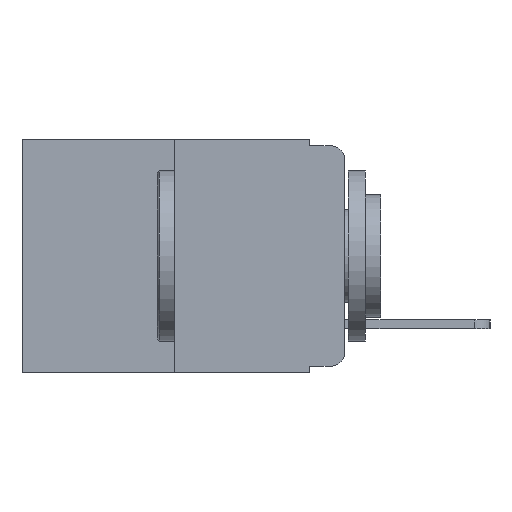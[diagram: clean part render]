
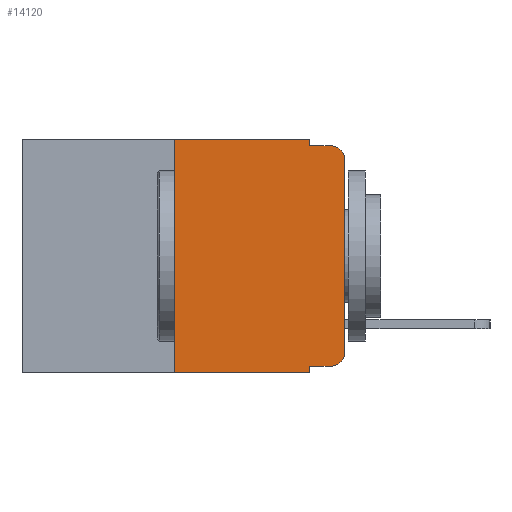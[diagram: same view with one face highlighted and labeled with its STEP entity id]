
A CAD part, left-side view. The second image highlights one B-rep face of the part: STEP entity #14120.
In plain terms, the highlighted planar face has unit normal (-1, 0, 0).
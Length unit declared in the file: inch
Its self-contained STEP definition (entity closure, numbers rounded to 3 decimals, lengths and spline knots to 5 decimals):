
#220 = AXIS2_PLACEMENT_3D ( 'NONE', #4102, #19524, #14592 ) ;
#433 = EDGE_LOOP ( 'NONE', ( #13091, #13113, #14780, #15248, #15609, #15630, #15636, #15817, #17762, #18595 ) ) ;
#1052 = VECTOR ( 'NONE', #4114, 39.37008 ) ;
#1091 = LINE ( 'NONE', #9057, #9512 ) ;
#1146 = CARTESIAN_POINT ( 'NONE',  ( 0., 0.25, -0.343 ) ) ;
#1528 = CIRCLE ( 'NONE', #2334, 0.02 ) ;
#1837 = CARTESIAN_POINT ( 'NONE',  ( 0., 0.051, 0. ) ) ;
#1863 = CARTESIAN_POINT ( 'NONE',  ( 0., 0., -0.03 ) ) ;
#1942 = LINE ( 'NONE', #18337, #5349 ) ;
#1950 = VERTEX_POINT ( 'NONE', #1146 ) ;
#2334 = AXIS2_PLACEMENT_3D ( 'NONE', #9263, #20120, #10343 ) ;
#3716 = EDGE_CURVE ( 'NONE', #14727, #7872, #1528, .T. ) ;
#3722 = DIRECTION ( 'NONE',  ( 0., 0., 1. ) ) ;
#3765 = CARTESIAN_POINT ( 'NONE',  ( 0., 0.02, -0.03 ) ) ;
#4102 = CARTESIAN_POINT ( 'NONE',  ( 0., 0.473, 0. ) ) ;
#4114 = DIRECTION ( 'NONE',  ( 0., -1., 0. ) ) ;
#4340 = DIRECTION ( 'NONE',  ( 0., 0., 1. ) ) ;
#4721 = FACE_OUTER_BOUND ( 'NONE', #433, .T. ) ;
#5335 = VECTOR ( 'NONE', #20934, 39.37008 ) ;
#5349 = VECTOR ( 'NONE', #21442, 39.37008 ) ;
#5462 = DIRECTION ( 'NONE',  ( 0., 0., -1. ) ) ;
#5794 = VERTEX_POINT ( 'NONE', #7338 ) ;
#5984 = EDGE_CURVE ( 'NONE', #5794, #14727, #1942, .T. ) ;
#7113 = EDGE_CURVE ( 'NONE', #5794, #13828, #18581, .T. ) ;
#7292 = DIRECTION ( 'NONE',  ( 0., -1., 0. ) ) ;
#7338 = CARTESIAN_POINT ( 'NONE',  ( 0., 0.051, -0.333 ) ) ;
#7716 = EDGE_CURVE ( 'NONE', #17515, #17455, #20288, .T. ) ;
#7872 = VERTEX_POINT ( 'NONE', #10326 ) ;
#8249 = EDGE_CURVE ( 'NONE', #1950, #17515, #1091, .T. ) ;
#8322 = LINE ( 'NONE', #14143, #16619 ) ;
#8709 = CARTESIAN_POINT ( 'NONE',  ( 0., 0.473, 0. ) ) ;
#9057 = CARTESIAN_POINT ( 'NONE',  ( 0., 0.25, 0. ) ) ;
#9191 = PLANE ( 'NONE',  #220 ) ;
#9263 = CARTESIAN_POINT ( 'NONE',  ( 0., 0.02, -0.313 ) ) ;
#9285 = VECTOR ( 'NONE', #3722, 39.37008 ) ;
#9380 = EDGE_CURVE ( 'NONE', #17455, #13485, #13062, .T. ) ;
#9401 = DIRECTION ( 'NONE',  ( 0., 0., -1. ) ) ;
#9512 = VECTOR ( 'NONE', #4340, 39.37008 ) ;
#10326 = CARTESIAN_POINT ( 'NONE',  ( 0., 0., -0.313 ) ) ;
#10343 = DIRECTION ( 'NONE',  ( 0., 0., -1. ) ) ;
#10504 = EDGE_CURVE ( 'NONE', #13485, #17508, #8322, .T. ) ;
#11599 = EDGE_CURVE ( 'NONE', #18146, #17508, #17863, .T. ) ;
#11746 = CARTESIAN_POINT ( 'NONE',  ( 0., 0.051, -0.343 ) ) ;
#11927 = CARTESIAN_POINT ( 'NONE',  ( 0., 0.02, -0.01 ) ) ;
#12545 = DIRECTION ( 'NONE',  ( 0., -1., 0. ) ) ;
#12707 = EDGE_CURVE ( 'NONE', #7872, #18146, #18064, .T. ) ;
#12728 = CARTESIAN_POINT ( 'NONE',  ( 0., 0.051, 0. ) ) ;
#13062 = LINE ( 'NONE', #12728, #21176 ) ;
#13091 = ORIENTED_EDGE ( 'NONE', *, *, #12707, .T. ) ;
#13113 = ORIENTED_EDGE ( 'NONE', *, *, #11599, .T. ) ;
#13485 = VERTEX_POINT ( 'NONE', #14015 ) ;
#13753 = CARTESIAN_POINT ( 'NONE',  ( 0., 0., 0. ) ) ;
#13828 = VERTEX_POINT ( 'NONE', #11746 ) ;
#14015 = CARTESIAN_POINT ( 'NONE',  ( 0., 0.051, -0.01 ) ) ;
#14120 = ADVANCED_FACE ( 'NONE', ( #4721 ), #9191, .F. ) ;
#14143 = CARTESIAN_POINT ( 'NONE',  ( 0., 0.051, -0.01 ) ) ;
#14400 = LINE ( 'NONE', #20592, #1052 ) ;
#14537 = AXIS2_PLACEMENT_3D ( 'NONE', #3765, #15445, #5462 ) ;
#14592 = DIRECTION ( 'NONE',  ( 0., 0., -1. ) ) ;
#14727 = VERTEX_POINT ( 'NONE', #19425 ) ;
#14780 = ORIENTED_EDGE ( 'NONE', *, *, #10504, .F. ) ;
#15020 = CARTESIAN_POINT ( 'NONE',  ( 0., 0.051, 0. ) ) ;
#15248 = ORIENTED_EDGE ( 'NONE', *, *, #9380, .F. ) ;
#15445 = DIRECTION ( 'NONE',  ( -1., 0., 0. ) ) ;
#15609 = ORIENTED_EDGE ( 'NONE', *, *, #7716, .F. ) ;
#15630 = ORIENTED_EDGE ( 'NONE', *, *, #8249, .F. ) ;
#15636 = ORIENTED_EDGE ( 'NONE', *, *, #18884, .T. ) ;
#15817 = ORIENTED_EDGE ( 'NONE', *, *, #7113, .F. ) ;
#16619 = VECTOR ( 'NONE', #12545, 39.37008 ) ;
#17455 = VERTEX_POINT ( 'NONE', #15020 ) ;
#17508 = VERTEX_POINT ( 'NONE', #11927 ) ;
#17515 = VERTEX_POINT ( 'NONE', #19990 ) ;
#17762 = ORIENTED_EDGE ( 'NONE', *, *, #5984, .T. ) ;
#17863 = CIRCLE ( 'NONE', #14537, 0.02 ) ;
#18064 = LINE ( 'NONE', #13753, #9285 ) ;
#18146 = VERTEX_POINT ( 'NONE', #1863 ) ;
#18337 = CARTESIAN_POINT ( 'NONE',  ( 0., 0.051, -0.333 ) ) ;
#18581 = LINE ( 'NONE', #1837, #5335 ) ;
#18595 = ORIENTED_EDGE ( 'NONE', *, *, #3716, .T. ) ;
#18884 = EDGE_CURVE ( 'NONE', #1950, #13828, #14400, .T. ) ;
#19425 = CARTESIAN_POINT ( 'NONE',  ( 0., 0.02, -0.333 ) ) ;
#19524 = DIRECTION ( 'NONE',  ( 1., 0., 0. ) ) ;
#19786 = VECTOR ( 'NONE', #7292, 39.37008 ) ;
#19990 = CARTESIAN_POINT ( 'NONE',  ( 0., 0.25, 0. ) ) ;
#20120 = DIRECTION ( 'NONE',  ( -1., 0., 0. ) ) ;
#20288 = LINE ( 'NONE', #8709, #19786 ) ;
#20592 = CARTESIAN_POINT ( 'NONE',  ( 0., 0.473, -0.343 ) ) ;
#20934 = DIRECTION ( 'NONE',  ( 0., 0., -1. ) ) ;
#21176 = VECTOR ( 'NONE', #9401, 39.37008 ) ;
#21442 = DIRECTION ( 'NONE',  ( 0., -1., 0. ) ) ;
